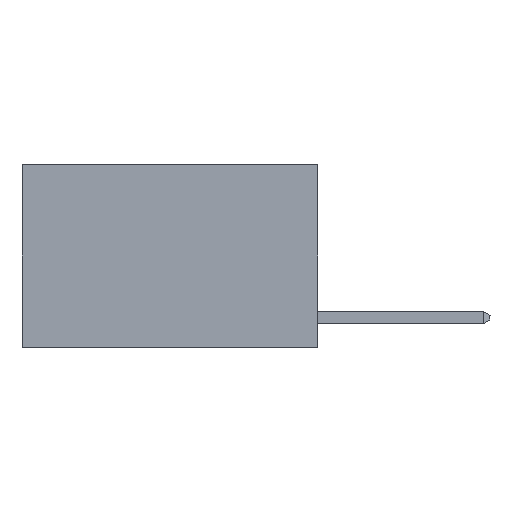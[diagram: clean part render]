
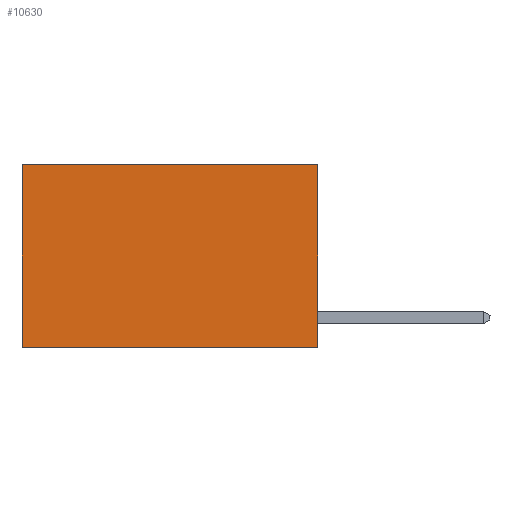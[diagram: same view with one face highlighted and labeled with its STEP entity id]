
A CAD part, left-side view. The second image highlights one B-rep face of the part: STEP entity #10630.
In plain terms, the highlighted planar face has unit normal (-1, 0, 0).
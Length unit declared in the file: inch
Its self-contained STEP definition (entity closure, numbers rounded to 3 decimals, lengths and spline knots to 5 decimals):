
#618 = CARTESIAN_POINT ( 'NONE',  ( 0.2625, 0., 0. ) ) ;
#1061 = EDGE_CURVE ( 'NONE', #1752, #4511, #18631, .T. ) ;
#1752 = VERTEX_POINT ( 'NONE', #8611 ) ;
#4511 = VERTEX_POINT ( 'NONE', #19574 ) ;
#4580 = LINE ( 'NONE', #6383, #7955 ) ;
#5130 = VERTEX_POINT ( 'NONE', #13574 ) ;
#5697 = EDGE_CURVE ( 'NONE', #13381, #1752, #7775, .T. ) ;
#6383 = CARTESIAN_POINT ( 'NONE',  ( 0.2625, 0.6, 0. ) ) ;
#7775 = LINE ( 'NONE', #618, #17659 ) ;
#7955 = VECTOR ( 'NONE', #14983, 39.37008 ) ;
#8098 = FACE_OUTER_BOUND ( 'NONE', #12004, .T. ) ;
#8611 = CARTESIAN_POINT ( 'NONE',  ( 0.2625, 0., -0.37 ) ) ;
#8744 = EDGE_CURVE ( 'NONE', #13381, #5130, #11396, .T. ) ;
#8838 = ORIENTED_EDGE ( 'NONE', *, *, #9384, .T. ) ;
#9262 = CARTESIAN_POINT ( 'NONE',  ( 0.2625, 0., 0. ) ) ;
#9384 = EDGE_CURVE ( 'NONE', #5130, #4511, #4580, .T. ) ;
#10127 = CARTESIAN_POINT ( 'NONE',  ( 0.2625, 0., -0.37 ) ) ;
#10630 = ADVANCED_FACE ( 'NONE', ( #8098 ), #13291, .F. ) ;
#11396 = LINE ( 'NONE', #9262, #18573 ) ;
#11708 = DIRECTION ( 'NONE',  ( 1., 0., 0. ) ) ;
#12004 = EDGE_LOOP ( 'NONE', ( #8838, #14665, #12017, #15190 ) ) ;
#12017 = ORIENTED_EDGE ( 'NONE', *, *, #5697, .F. ) ;
#13291 = PLANE ( 'NONE',  #14369 ) ;
#13381 = VERTEX_POINT ( 'NONE', #19406 ) ;
#13574 = CARTESIAN_POINT ( 'NONE',  ( 0.2625, 0.6, 0. ) ) ;
#14369 = AXIS2_PLACEMENT_3D ( 'NONE', #20334, #11708, #20222 ) ;
#14665 = ORIENTED_EDGE ( 'NONE', *, *, #1061, .F. ) ;
#14983 = DIRECTION ( 'NONE',  ( 0., 0., -1. ) ) ;
#15190 = ORIENTED_EDGE ( 'NONE', *, *, #8744, .T. ) ;
#16266 = DIRECTION ( 'NONE',  ( 0., 0., -1. ) ) ;
#16573 = VECTOR ( 'NONE', #22362, 39.37008 ) ;
#17659 = VECTOR ( 'NONE', #16266, 39.37008 ) ;
#18573 = VECTOR ( 'NONE', #20130, 39.37008 ) ;
#18631 = LINE ( 'NONE', #10127, #16573 ) ;
#19406 = CARTESIAN_POINT ( 'NONE',  ( 0.2625, 0., 0. ) ) ;
#19574 = CARTESIAN_POINT ( 'NONE',  ( 0.2625, 0.6, -0.37 ) ) ;
#20130 = DIRECTION ( 'NONE',  ( 0., 1., 0. ) ) ;
#20222 = DIRECTION ( 'NONE',  ( 0., 0., -1. ) ) ;
#20334 = CARTESIAN_POINT ( 'NONE',  ( 0.2625, 0., 0. ) ) ;
#22362 = DIRECTION ( 'NONE',  ( 0., 1., 0. ) ) ;
